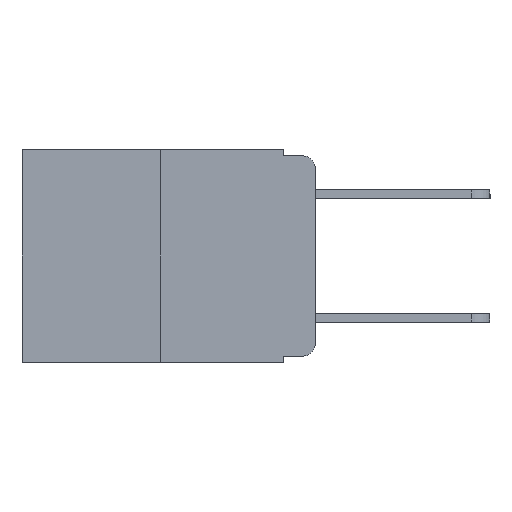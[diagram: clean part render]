
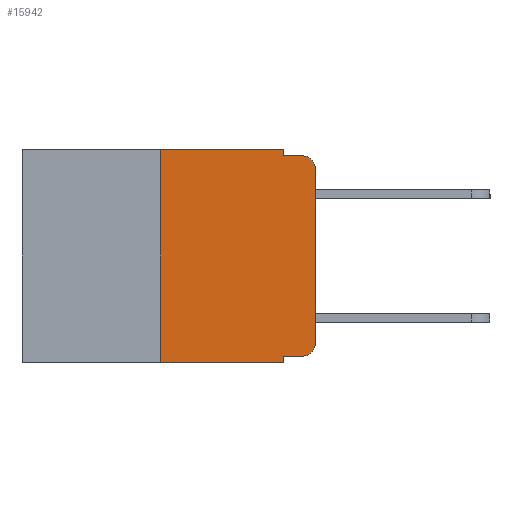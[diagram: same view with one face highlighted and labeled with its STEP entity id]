
A CAD part, left-side view. The second image highlights one B-rep face of the part: STEP entity #15942.
In plain terms, the highlighted planar face has unit normal (-1, 0, 0).
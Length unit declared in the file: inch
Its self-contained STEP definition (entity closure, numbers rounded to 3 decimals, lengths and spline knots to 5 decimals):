
#136 = EDGE_CURVE ( 'NONE', #10376, #17975, #18702, .T. ) ;
#278 = LINE ( 'NONE', #17633, #13087 ) ;
#1166 = DIRECTION ( 'NONE',  ( 0., 0., -1. ) ) ;
#1378 = DIRECTION ( 'NONE',  ( 0., -1., 0. ) ) ;
#1570 = ORIENTED_EDGE ( 'NONE', *, *, #2273, .T. ) ;
#1875 = ORIENTED_EDGE ( 'NONE', *, *, #17370, .F. ) ;
#2029 = AXIS2_PLACEMENT_3D ( 'NONE', #17214, #18856, #8960 ) ;
#2103 = VERTEX_POINT ( 'NONE', #5437 ) ;
#2273 = EDGE_CURVE ( 'NONE', #20637, #5188, #10628, .T. ) ;
#2646 = CARTESIAN_POINT ( 'NONE',  ( 0., 0.25, 0. ) ) ;
#3289 = VECTOR ( 'NONE', #5670, 39.37008 ) ;
#3904 = ORIENTED_EDGE ( 'NONE', *, *, #136, .T. ) ;
#4220 = ORIENTED_EDGE ( 'NONE', *, *, #14221, .F. ) ;
#4356 = LINE ( 'NONE', #19334, #12726 ) ;
#4439 = CARTESIAN_POINT ( 'NONE',  ( 0., 0.02, -0.03 ) ) ;
#5188 = VERTEX_POINT ( 'NONE', #11079 ) ;
#5263 = VECTOR ( 'NONE', #12670, 39.37008 ) ;
#5408 = EDGE_CURVE ( 'NONE', #21065, #20637, #15926, .T. ) ;
#5437 = CARTESIAN_POINT ( 'NONE',  ( 0., 0.051, 0. ) ) ;
#5670 = DIRECTION ( 'NONE',  ( 0., 0., 1. ) ) ;
#6028 = EDGE_CURVE ( 'NONE', #14911, #17975, #18014, .T. ) ;
#6563 = ORIENTED_EDGE ( 'NONE', *, *, #5408, .T. ) ;
#6641 = VECTOR ( 'NONE', #9476, 39.37008 ) ;
#6763 = EDGE_CURVE ( 'NONE', #7025, #7243, #14827, .T. ) ;
#7025 = VERTEX_POINT ( 'NONE', #8705 ) ;
#7243 = VERTEX_POINT ( 'NONE', #13896 ) ;
#7783 = LINE ( 'NONE', #13940, #3289 ) ;
#8705 = CARTESIAN_POINT ( 'NONE',  ( 0., 0.25, -0.343 ) ) ;
#8960 = DIRECTION ( 'NONE',  ( 0., 0., -1. ) ) ;
#9476 = DIRECTION ( 'NONE',  ( 0., 0., 1. ) ) ;
#9786 = CARTESIAN_POINT ( 'NONE',  ( 0., 0.051, -0.333 ) ) ;
#9885 = VERTEX_POINT ( 'NONE', #19423 ) ;
#10376 = VERTEX_POINT ( 'NONE', #10942 ) ;
#10628 = CIRCLE ( 'NONE', #20314, 0.02 ) ;
#10942 = CARTESIAN_POINT ( 'NONE',  ( 0., 0., -0.03 ) ) ;
#11010 = VECTOR ( 'NONE', #1378, 39.37008 ) ;
#11059 = LINE ( 'NONE', #2646, #6641 ) ;
#11079 = CARTESIAN_POINT ( 'NONE',  ( 0., 0., -0.313 ) ) ;
#11265 = EDGE_CURVE ( 'NONE', #21065, #7243, #19708, .T. ) ;
#11284 = CARTESIAN_POINT ( 'NONE',  ( 0., 0.02, -0.333 ) ) ;
#11981 = DIRECTION ( 'NONE',  ( 0., -1., 0. ) ) ;
#12385 = CARTESIAN_POINT ( 'NONE',  ( 0., 0.051, -0.01 ) ) ;
#12631 = ORIENTED_EDGE ( 'NONE', *, *, #11265, .F. ) ;
#12670 = DIRECTION ( 'NONE',  ( 0., -1., 0. ) ) ;
#12726 = VECTOR ( 'NONE', #21028, 39.37008 ) ;
#13078 = ORIENTED_EDGE ( 'NONE', *, *, #13620, .F. ) ;
#13087 = VECTOR ( 'NONE', #16034, 39.37008 ) ;
#13555 = ORIENTED_EDGE ( 'NONE', *, *, #17868, .T. ) ;
#13620 = EDGE_CURVE ( 'NONE', #7025, #9885, #11059, .T. ) ;
#13896 = CARTESIAN_POINT ( 'NONE',  ( 0., 0.051, -0.343 ) ) ;
#13940 = CARTESIAN_POINT ( 'NONE',  ( 0., 0., 0. ) ) ;
#14221 = EDGE_CURVE ( 'NONE', #2103, #14911, #278, .T. ) ;
#14827 = LINE ( 'NONE', #18656, #18740 ) ;
#14911 = VERTEX_POINT ( 'NONE', #19320 ) ;
#15290 = VECTOR ( 'NONE', #1166, 39.37008 ) ;
#15408 = AXIS2_PLACEMENT_3D ( 'NONE', #4439, #20666, #16929 ) ;
#15510 = PLANE ( 'NONE',  #2029 ) ;
#15596 = FACE_OUTER_BOUND ( 'NONE', #17520, .T. ) ;
#15821 = CARTESIAN_POINT ( 'NONE',  ( 0., 0.051, -0.333 ) ) ;
#15918 = CARTESIAN_POINT ( 'NONE',  ( 0., 0.02, -0.01 ) ) ;
#15926 = LINE ( 'NONE', #9786, #11010 ) ;
#15942 = ADVANCED_FACE ( 'NONE', ( #15596 ), #15510, .F. ) ;
#16034 = DIRECTION ( 'NONE',  ( 0., 0., -1. ) ) ;
#16119 = DIRECTION ( 'NONE',  ( 0., 0., -1. ) ) ;
#16918 = CARTESIAN_POINT ( 'NONE',  ( 0., 0.02, -0.313 ) ) ;
#16929 = DIRECTION ( 'NONE',  ( 0., 0., -1. ) ) ;
#17063 = DIRECTION ( 'NONE',  ( -1., 0., 0. ) ) ;
#17214 = CARTESIAN_POINT ( 'NONE',  ( 0., 0.473, 0. ) ) ;
#17370 = EDGE_CURVE ( 'NONE', #9885, #2103, #4356, .T. ) ;
#17520 = EDGE_LOOP ( 'NONE', ( #13555, #3904, #17570, #4220, #1875, #13078, #18304, #12631, #6563, #1570 ) ) ;
#17570 = ORIENTED_EDGE ( 'NONE', *, *, #6028, .F. ) ;
#17633 = CARTESIAN_POINT ( 'NONE',  ( 0., 0.051, 0. ) ) ;
#17868 = EDGE_CURVE ( 'NONE', #5188, #10376, #7783, .T. ) ;
#17975 = VERTEX_POINT ( 'NONE', #15918 ) ;
#18014 = LINE ( 'NONE', #12385, #5263 ) ;
#18304 = ORIENTED_EDGE ( 'NONE', *, *, #6763, .T. ) ;
#18656 = CARTESIAN_POINT ( 'NONE',  ( 0., 0.473, -0.343 ) ) ;
#18702 = CIRCLE ( 'NONE', #15408, 0.02 ) ;
#18740 = VECTOR ( 'NONE', #11981, 39.37008 ) ;
#18856 = DIRECTION ( 'NONE',  ( 1., 0., 0. ) ) ;
#19320 = CARTESIAN_POINT ( 'NONE',  ( 0., 0.051, -0.01 ) ) ;
#19334 = CARTESIAN_POINT ( 'NONE',  ( 0., 0.473, 0. ) ) ;
#19423 = CARTESIAN_POINT ( 'NONE',  ( 0., 0.25, 0. ) ) ;
#19708 = LINE ( 'NONE', #21155, #15290 ) ;
#20314 = AXIS2_PLACEMENT_3D ( 'NONE', #16918, #17063, #16119 ) ;
#20637 = VERTEX_POINT ( 'NONE', #11284 ) ;
#20666 = DIRECTION ( 'NONE',  ( -1., 0., 0. ) ) ;
#21028 = DIRECTION ( 'NONE',  ( 0., -1., 0. ) ) ;
#21065 = VERTEX_POINT ( 'NONE', #15821 ) ;
#21155 = CARTESIAN_POINT ( 'NONE',  ( 0., 0.051, 0. ) ) ;
